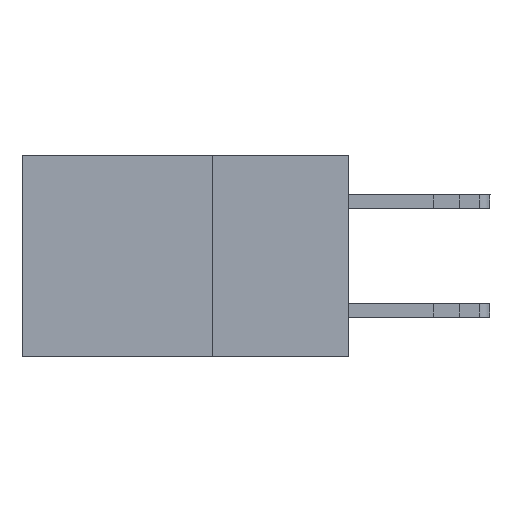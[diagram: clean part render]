
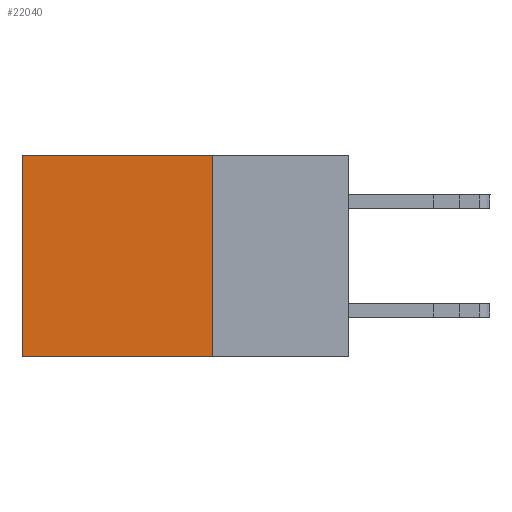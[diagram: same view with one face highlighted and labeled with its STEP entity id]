
A CAD part, left-side view. The second image highlights one B-rep face of the part: STEP entity #22040.
In plain terms, the highlighted planar face has unit normal (-1, 0, 0).
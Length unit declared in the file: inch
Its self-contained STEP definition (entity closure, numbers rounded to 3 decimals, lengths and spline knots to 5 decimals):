
#271 = VECTOR ( 'NONE', #28286, 39.37008 ) ;
#719 = CARTESIAN_POINT ( 'NONE',  ( 0.298, 0.25, 0. ) ) ;
#858 = EDGE_LOOP ( 'NONE', ( #28310, #6974, #12756, #4484 ) ) ;
#1717 = EDGE_CURVE ( 'NONE', #27838, #23737, #9068, .T. ) ;
#4484 = ORIENTED_EDGE ( 'NONE', *, *, #1717, .T. ) ;
#5145 = DIRECTION ( 'NONE',  ( 0., 1., 0. ) ) ;
#6145 = VERTEX_POINT ( 'NONE', #26108 ) ;
#6413 = CARTESIAN_POINT ( 'NONE',  ( 0.298, 0.25, -0.37 ) ) ;
#6580 = LINE ( 'NONE', #13797, #9374 ) ;
#6974 = ORIENTED_EDGE ( 'NONE', *, *, #13840, .F. ) ;
#7052 = VECTOR ( 'NONE', #5145, 39.37008 ) ;
#9068 = LINE ( 'NONE', #27158, #7052 ) ;
#9374 = VECTOR ( 'NONE', #20172, 39.37008 ) ;
#9871 = DIRECTION ( 'NONE',  ( 0., 0., -1. ) ) ;
#10751 = CARTESIAN_POINT ( 'NONE',  ( 0.298, 0.25, -0.37 ) ) ;
#10821 = VERTEX_POINT ( 'NONE', #6413 ) ;
#12341 = AXIS2_PLACEMENT_3D ( 'NONE', #18717, #16255, #9871 ) ;
#12756 = ORIENTED_EDGE ( 'NONE', *, *, #28221, .F. ) ;
#13349 = FACE_OUTER_BOUND ( 'NONE', #858, .T. ) ;
#13797 = CARTESIAN_POINT ( 'NONE',  ( 0.298, 0.6, 0. ) ) ;
#13840 = EDGE_CURVE ( 'NONE', #10821, #6145, #21735, .T. ) ;
#16255 = DIRECTION ( 'NONE',  ( 1., 0., 0. ) ) ;
#18717 = CARTESIAN_POINT ( 'NONE',  ( 0.298, 0.25, 0. ) ) ;
#19475 = CARTESIAN_POINT ( 'NONE',  ( 0.298, 0.25, 0. ) ) ;
#19577 = DIRECTION ( 'NONE',  ( 0., 1., 0. ) ) ;
#20172 = DIRECTION ( 'NONE',  ( 0., 0., -1. ) ) ;
#21643 = LINE ( 'NONE', #19475, #271 ) ;
#21735 = LINE ( 'NONE', #10751, #22746 ) ;
#22040 = ADVANCED_FACE ( 'NONE', ( #13349 ), #27387, .F. ) ;
#22746 = VECTOR ( 'NONE', #19577, 39.37008 ) ;
#23340 = CARTESIAN_POINT ( 'NONE',  ( 0.298, 0.6, 0. ) ) ;
#23535 = EDGE_CURVE ( 'NONE', #23737, #6145, #6580, .T. ) ;
#23737 = VERTEX_POINT ( 'NONE', #23340 ) ;
#26108 = CARTESIAN_POINT ( 'NONE',  ( 0.298, 0.6, -0.37 ) ) ;
#27158 = CARTESIAN_POINT ( 'NONE',  ( 0.298, 0.25, 0. ) ) ;
#27387 = PLANE ( 'NONE',  #12341 ) ;
#27838 = VERTEX_POINT ( 'NONE', #719 ) ;
#28221 = EDGE_CURVE ( 'NONE', #27838, #10821, #21643, .T. ) ;
#28286 = DIRECTION ( 'NONE',  ( 0., 0., -1. ) ) ;
#28310 = ORIENTED_EDGE ( 'NONE', *, *, #23535, .T. ) ;
